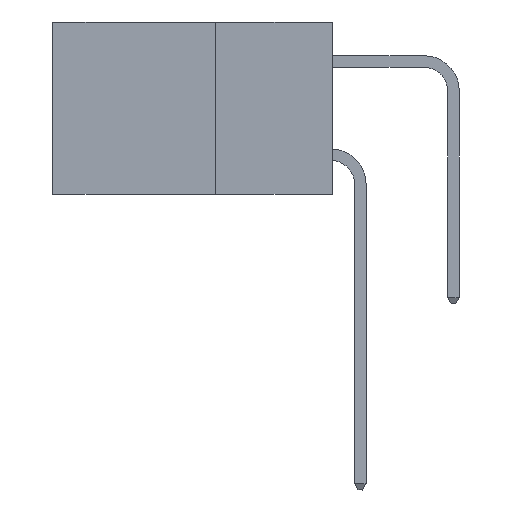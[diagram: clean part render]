
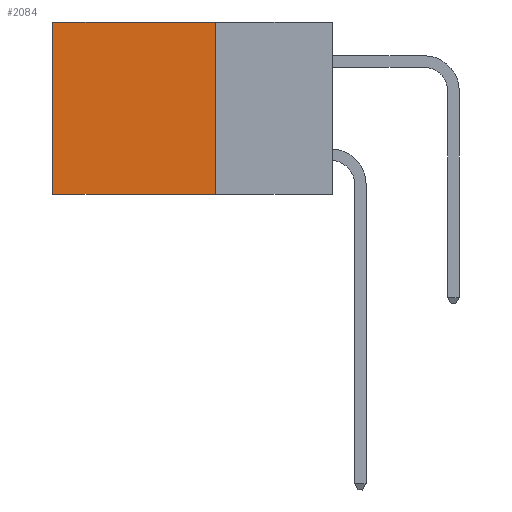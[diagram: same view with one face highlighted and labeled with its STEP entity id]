
A CAD part, left-side view. The second image highlights one B-rep face of the part: STEP entity #2084.
In plain terms, the highlighted planar face has unit normal (-1, 0, 0).
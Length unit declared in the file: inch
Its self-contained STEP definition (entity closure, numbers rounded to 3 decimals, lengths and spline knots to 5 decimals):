
#240 = VERTEX_POINT ( 'NONE', #2632 ) ;
#410 = CARTESIAN_POINT ( 'NONE',  ( 0.298, 0.25, 0. ) ) ;
#1054 = DIRECTION ( 'NONE',  ( 0., 1., 0. ) ) ;
#1093 = DIRECTION ( 'NONE',  ( 0., 0., -1. ) ) ;
#1221 = VECTOR ( 'NONE', #7117, 39.37008 ) ;
#1455 = FACE_OUTER_BOUND ( 'NONE', #3218, .T. ) ;
#1944 = LINE ( 'NONE', #9029, #11038 ) ;
#2084 = ADVANCED_FACE ( 'NONE', ( #1455 ), #2199, .F. ) ;
#2188 = LINE ( 'NONE', #9284, #5933 ) ;
#2199 = PLANE ( 'NONE',  #3253 ) ;
#2632 = CARTESIAN_POINT ( 'NONE',  ( 0.298, 0.25, -0.37 ) ) ;
#3218 = EDGE_LOOP ( 'NONE', ( #8306, #10212, #7860, #8090 ) ) ;
#3253 = AXIS2_PLACEMENT_3D ( 'NONE', #4059, #7100, #1093 ) ;
#3264 = LINE ( 'NONE', #9259, #5468 ) ;
#3280 = DIRECTION ( 'NONE',  ( 0., 0., -1. ) ) ;
#3896 = LINE ( 'NONE', #8258, #1221 ) ;
#3920 = VERTEX_POINT ( 'NONE', #8050 ) ;
#4059 = CARTESIAN_POINT ( 'NONE',  ( 0.298, 0.25, 0. ) ) ;
#5468 = VECTOR ( 'NONE', #9157, 39.37008 ) ;
#5730 = VERTEX_POINT ( 'NONE', #410 ) ;
#5933 = VECTOR ( 'NONE', #3280, 39.37008 ) ;
#6073 = EDGE_CURVE ( 'NONE', #6719, #3920, #2188, .T. ) ;
#6719 = VERTEX_POINT ( 'NONE', #6941 ) ;
#6941 = CARTESIAN_POINT ( 'NONE',  ( 0.298, 0.6, 0. ) ) ;
#7100 = DIRECTION ( 'NONE',  ( 1., 0., 0. ) ) ;
#7117 = DIRECTION ( 'NONE',  ( 0., 1., 0. ) ) ;
#7860 = ORIENTED_EDGE ( 'NONE', *, *, #11711, .F. ) ;
#8050 = CARTESIAN_POINT ( 'NONE',  ( 0.298, 0.6, -0.37 ) ) ;
#8090 = ORIENTED_EDGE ( 'NONE', *, *, #11699, .T. ) ;
#8258 = CARTESIAN_POINT ( 'NONE',  ( 0.298, 0.25, 0. ) ) ;
#8306 = ORIENTED_EDGE ( 'NONE', *, *, #6073, .T. ) ;
#9029 = CARTESIAN_POINT ( 'NONE',  ( 0.298, 0.25, -0.37 ) ) ;
#9157 = DIRECTION ( 'NONE',  ( 0., 0., -1. ) ) ;
#9259 = CARTESIAN_POINT ( 'NONE',  ( 0.298, 0.25, 0. ) ) ;
#9284 = CARTESIAN_POINT ( 'NONE',  ( 0.298, 0.6, 0. ) ) ;
#9378 = EDGE_CURVE ( 'NONE', #240, #3920, #1944, .T. ) ;
#10212 = ORIENTED_EDGE ( 'NONE', *, *, #9378, .F. ) ;
#11038 = VECTOR ( 'NONE', #1054, 39.37008 ) ;
#11699 = EDGE_CURVE ( 'NONE', #5730, #6719, #3896, .T. ) ;
#11711 = EDGE_CURVE ( 'NONE', #5730, #240, #3264, .T. ) ;
